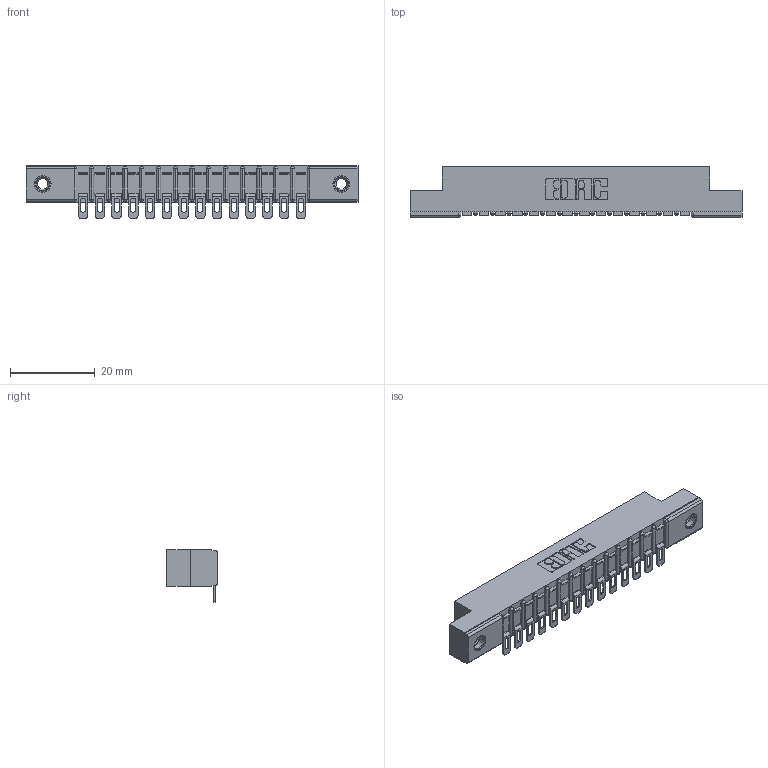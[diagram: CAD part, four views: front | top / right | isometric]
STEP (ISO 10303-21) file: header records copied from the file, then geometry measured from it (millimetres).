
FILE_DESCRIPTION (( 'STEP AP203' ), '1' );
FILE_NAME ('307-014-554-107.STEP', '2019-09-04T20:43:00', ( '' ), ( '' ), 'SwSTEP 2.0', 'SolidWorks 2016', '' );
FILE_SCHEMA (( 'CONFIG_CONTROL_DESIGN' ));
Length unit declared in the file: inch
Products named in the file (4): 307-014-554-107; 307 Part_.156 Dia Mounting Holes; 307-290-002_554; 345-250-001_345-250-005-103
Assembly tree (17 placements, depth 2):
  307-014-554-107
    307 Part_.156 Dia Mounting Holes
    307-290-002_554  x14
    345-250-001_345-250-005-103  x2
Bounding box: 78.49 x 12.01 x 12.52 mm (x, y, z)
Volume: 5168.8 mm3; surface area: 9049.6 mm2
Topology: 17 solids, 17 shells, 1327 faces, 4001 edges, 2618 vertices
Faces by surface type: plane 746, cylinder 535, sphere 30, cone 12, torus 4
Entity records: 17604 total; most frequent: CARTESIAN_POINT 2945, ORIENTED_EDGE 2928, DIRECTION 2890, EDGE_CURVE 1464, LINE 1100, VECTOR 1100, VERTEX_POINT 950, AXIS2_PLACEMENT_3D 895
